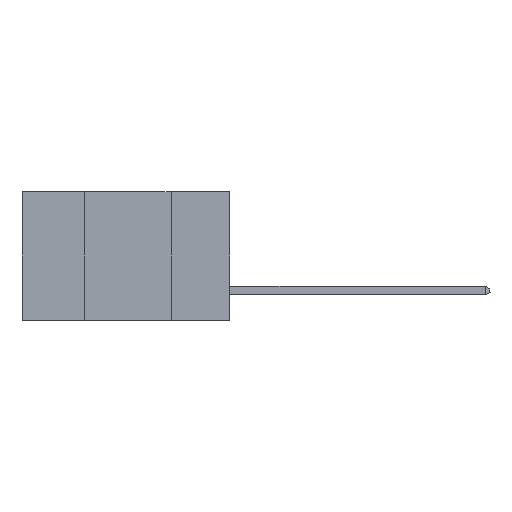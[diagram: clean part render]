
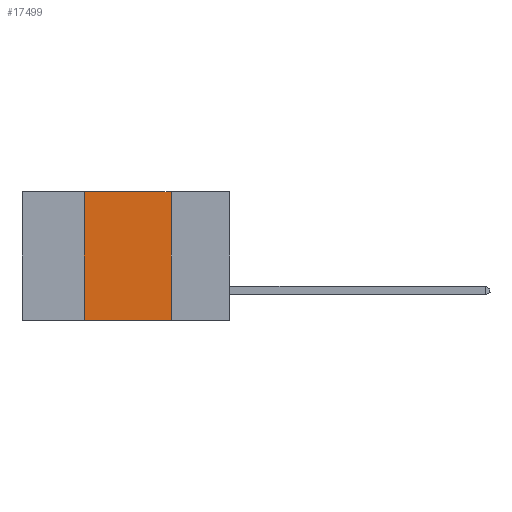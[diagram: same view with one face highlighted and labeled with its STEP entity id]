
A CAD part, left-side view. The second image highlights one B-rep face of the part: STEP entity #17499.
In plain terms, the highlighted planar face has unit normal (-1, 0, 0).
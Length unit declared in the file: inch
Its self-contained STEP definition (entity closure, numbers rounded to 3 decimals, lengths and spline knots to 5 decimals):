
#1305 = LINE ( 'NONE', #4933, #26014 ) ;
#1813 = DIRECTION ( 'NONE',  ( 1., 0., 0. ) ) ;
#2657 = AXIS2_PLACEMENT_3D ( 'NONE', #15335, #1813, #20535 ) ;
#3322 = VECTOR ( 'NONE', #20918, 39.37008 ) ;
#3562 = VECTOR ( 'NONE', #11123, 39.37008 ) ;
#4122 = VERTEX_POINT ( 'NONE', #13341 ) ;
#4933 = CARTESIAN_POINT ( 'NONE',  ( 0., 0.6, 0. ) ) ;
#5788 = ORIENTED_EDGE ( 'NONE', *, *, #17936, .F. ) ;
#6967 = EDGE_CURVE ( 'NONE', #4122, #18477, #17217, .T. ) ;
#7161 = LINE ( 'NONE', #18965, #3322 ) ;
#7400 = CARTESIAN_POINT ( 'NONE',  ( 0., 0.42, 0. ) ) ;
#11123 = DIRECTION ( 'NONE',  ( 0., 0., 1. ) ) ;
#11243 = CARTESIAN_POINT ( 'NONE',  ( 0., 0.17, -0.37 ) ) ;
#13341 = CARTESIAN_POINT ( 'NONE',  ( 0., 0.42, -0.37 ) ) ;
#14174 = VERTEX_POINT ( 'NONE', #15344 ) ;
#14186 = PLANE ( 'NONE',  #2657 ) ;
#14297 = ORIENTED_EDGE ( 'NONE', *, *, #20753, .F. ) ;
#14364 = FACE_OUTER_BOUND ( 'NONE', #24557, .T. ) ;
#14958 = DIRECTION ( 'NONE',  ( 0., -1., 0. ) ) ;
#15335 = CARTESIAN_POINT ( 'NONE',  ( 0., 0.6, 0. ) ) ;
#15344 = CARTESIAN_POINT ( 'NONE',  ( 0., 0.17, 0. ) ) ;
#16586 = EDGE_CURVE ( 'NONE', #4122, #20292, #7161, .T. ) ;
#17217 = LINE ( 'NONE', #7400, #3562 ) ;
#17499 = ADVANCED_FACE ( 'NONE', ( #14364 ), #14186, .F. ) ;
#17554 = LINE ( 'NONE', #26020, #18832 ) ;
#17936 = EDGE_CURVE ( 'NONE', #14174, #20292, #17554, .T. ) ;
#18477 = VERTEX_POINT ( 'NONE', #22123 ) ;
#18832 = VECTOR ( 'NONE', #19752, 39.37008 ) ;
#18965 = CARTESIAN_POINT ( 'NONE',  ( 0., 0.6, -0.37 ) ) ;
#19752 = DIRECTION ( 'NONE',  ( 0., 0., -1. ) ) ;
#20292 = VERTEX_POINT ( 'NONE', #11243 ) ;
#20535 = DIRECTION ( 'NONE',  ( 0., 0., -1. ) ) ;
#20753 = EDGE_CURVE ( 'NONE', #18477, #14174, #1305, .T. ) ;
#20918 = DIRECTION ( 'NONE',  ( 0., -1., 0. ) ) ;
#21717 = ORIENTED_EDGE ( 'NONE', *, *, #6967, .F. ) ;
#21864 = ORIENTED_EDGE ( 'NONE', *, *, #16586, .T. ) ;
#22123 = CARTESIAN_POINT ( 'NONE',  ( 0., 0.42, 0. ) ) ;
#24557 = EDGE_LOOP ( 'NONE', ( #5788, #14297, #21717, #21864 ) ) ;
#26014 = VECTOR ( 'NONE', #14958, 39.37008 ) ;
#26020 = CARTESIAN_POINT ( 'NONE',  ( 0., 0.17, 0. ) ) ;
